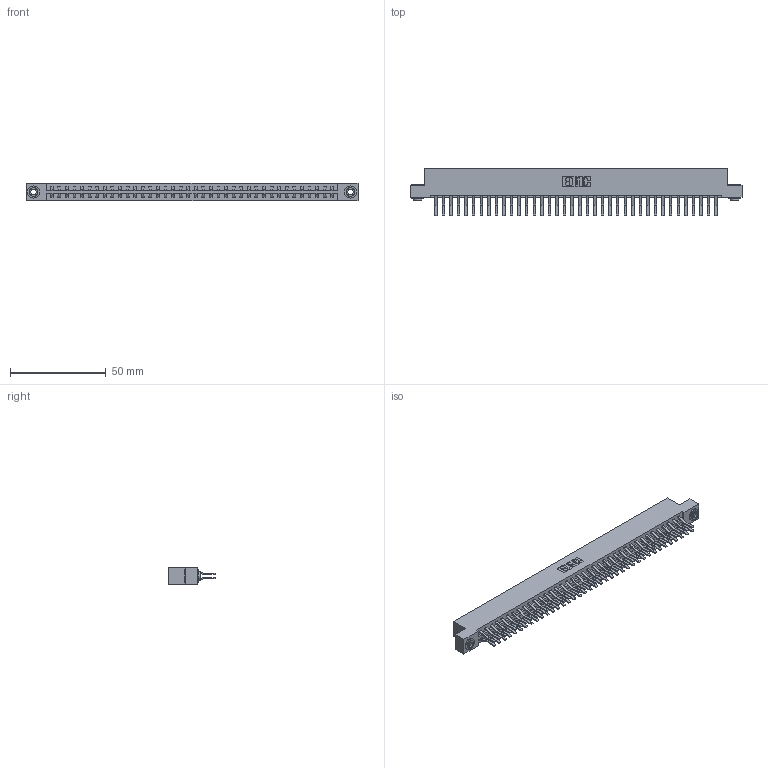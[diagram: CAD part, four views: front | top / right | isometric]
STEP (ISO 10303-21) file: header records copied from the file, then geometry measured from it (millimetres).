
FILE_DESCRIPTION (( 'STEP AP203' ), '1' );
FILE_NAME ('387-076-560-203.STEP', '2019-10-22T04:54:36', ( '' ), ( '' ), 'SwSTEP 2.0', 'SolidWorks 2016', '' );
FILE_SCHEMA (( 'CONFIG_CONTROL_DESIGN' ));
Length unit declared in the file: inch
Products named in the file (4): 345-250-002_345-250-002-102; 387-076-560-203; 345-292-001_560 Tail; 337 Part_Flush Mounting Lugs - 0.156 Dia-TH
Assembly tree (79 placements, depth 2):
  387-076-560-203
    337 Part_Flush Mounting Lugs - 0.156 Dia-TH
    345-292-001_560 Tail  x76
    345-250-002_345-250-002-102  x2
Bounding box: 173.58 x 24.78 x 9.4 mm (x, y, z)
Volume: 18757.9 mm3; surface area: 22833.2 mm2
Topology: 79 solids, 79 shells, 4408 faces, 13079 edges, 8614 vertices
Faces by surface type: plane 2968, cylinder 1432, cone 8
Entity records: 30718 total; most frequent: CARTESIAN_POINT 5153, ORIENTED_EDGE 5082, DIRECTION 4427, EDGE_CURVE 2541, LINE 2385, VECTOR 2385, VERTEX_POINT 1690, AXIS2_PLACEMENT_3D 1021
